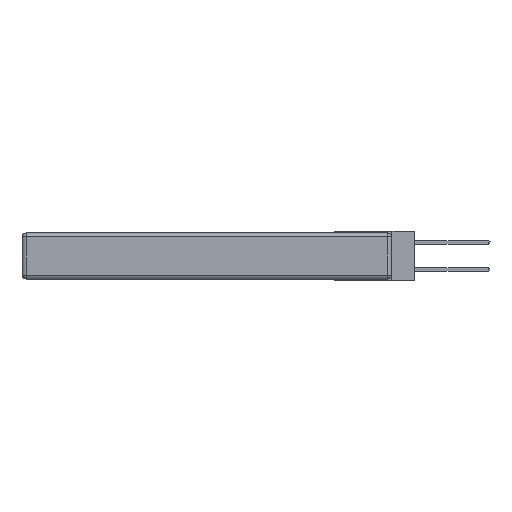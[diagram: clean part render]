
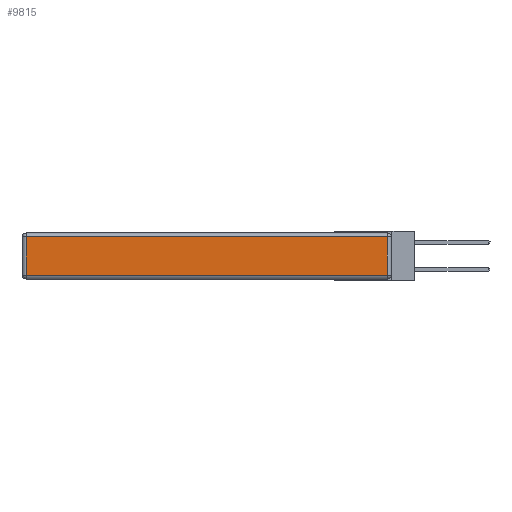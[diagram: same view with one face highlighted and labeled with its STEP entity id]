
A CAD part, left-side view. The second image highlights one B-rep face of the part: STEP entity #9815.
In plain terms, the highlighted planar face has unit normal (-1, 0, 0).
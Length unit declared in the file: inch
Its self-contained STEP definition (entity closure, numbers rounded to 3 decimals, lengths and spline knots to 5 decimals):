
#926 = EDGE_CURVE ( 'NONE', #16938, #23443, #32127, .T. ) ;
#1242 = CARTESIAN_POINT ( 'NONE',  ( 0., 0.03, -0.343 ) ) ;
#1496 = FACE_OUTER_BOUND ( 'NONE', #5493, .T. ) ;
#2431 = CARTESIAN_POINT ( 'NONE',  ( 0., 0.03, -0.313 ) ) ;
#3591 = CARTESIAN_POINT ( 'NONE',  ( 0., 0., -0.343 ) ) ;
#5016 = VERTEX_POINT ( 'NONE', #15480 ) ;
#5493 = EDGE_LOOP ( 'NONE', ( #10254, #13770, #7655, #7306 ) ) ;
#6666 = PLANE ( 'NONE',  #25112 ) ;
#7306 = ORIENTED_EDGE ( 'NONE', *, *, #18861, .T. ) ;
#7655 = ORIENTED_EDGE ( 'NONE', *, *, #9559, .T. ) ;
#8511 = VECTOR ( 'NONE', #16864, 39.37008 ) ;
#9174 = DIRECTION ( 'NONE',  ( 0., 1., 0. ) ) ;
#9559 = EDGE_CURVE ( 'NONE', #23443, #5016, #11793, .T. ) ;
#9815 = ADVANCED_FACE ( 'NONE', ( #1496 ), #6666, .T. ) ;
#10254 = ORIENTED_EDGE ( 'NONE', *, *, #23506, .T. ) ;
#11523 = DIRECTION ( 'NONE',  ( -1., 0., 0. ) ) ;
#11793 = LINE ( 'NONE', #24978, #27099 ) ;
#12365 = VECTOR ( 'NONE', #31369, 39.37008 ) ;
#13770 = ORIENTED_EDGE ( 'NONE', *, *, #926, .T. ) ;
#14392 = DIRECTION ( 'NONE',  ( 0., 0., 1. ) ) ;
#15480 = CARTESIAN_POINT ( 'NONE',  ( 0., 2.72, -0.03 ) ) ;
#15577 = VECTOR ( 'NONE', #16307, 39.37008 ) ;
#16307 = DIRECTION ( 'NONE',  ( 0., 0., -1. ) ) ;
#16864 = DIRECTION ( 'NONE',  ( 0., 0., 1. ) ) ;
#16938 = VERTEX_POINT ( 'NONE', #2431 ) ;
#18861 = EDGE_CURVE ( 'NONE', #5016, #30806, #20569, .T. ) ;
#19417 = LINE ( 'NONE', #34141, #12365 ) ;
#20569 = LINE ( 'NONE', #32346, #15577 ) ;
#23443 = VERTEX_POINT ( 'NONE', #33606 ) ;
#23506 = EDGE_CURVE ( 'NONE', #30806, #16938, #19417, .T. ) ;
#24978 = CARTESIAN_POINT ( 'NONE',  ( 0., 2.75, -0.03 ) ) ;
#25112 = AXIS2_PLACEMENT_3D ( 'NONE', #3591, #11523, #14392 ) ;
#27099 = VECTOR ( 'NONE', #9174, 39.37008 ) ;
#30806 = VERTEX_POINT ( 'NONE', #32576 ) ;
#31369 = DIRECTION ( 'NONE',  ( 0., -1., 0. ) ) ;
#32127 = LINE ( 'NONE', #1242, #8511 ) ;
#32346 = CARTESIAN_POINT ( 'NONE',  ( 0., 2.72, -0.343 ) ) ;
#32576 = CARTESIAN_POINT ( 'NONE',  ( 0., 2.72, -0.313 ) ) ;
#33606 = CARTESIAN_POINT ( 'NONE',  ( 0., 0.03, -0.03 ) ) ;
#34141 = CARTESIAN_POINT ( 'NONE',  ( 0., 0., -0.313 ) ) ;
